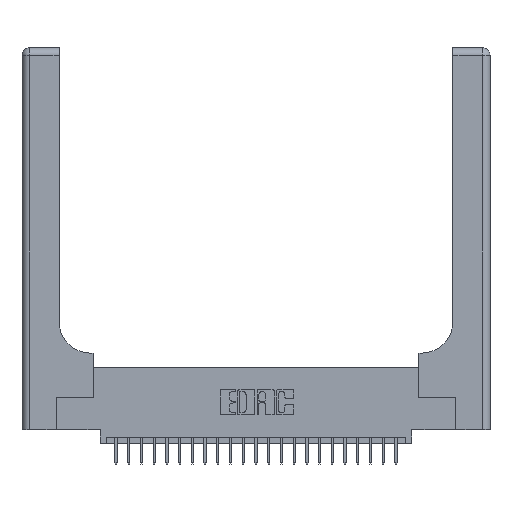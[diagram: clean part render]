
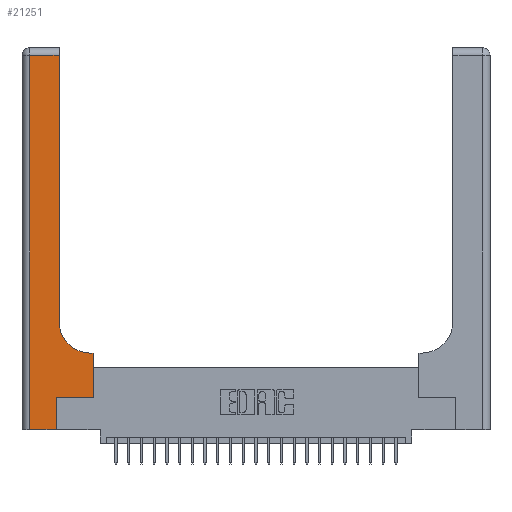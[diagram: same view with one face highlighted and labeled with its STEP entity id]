
A CAD part, top view. The second image highlights one B-rep face of the part: STEP entity #21251.
In plain terms, the highlighted planar face has unit normal (0, 0, 1).
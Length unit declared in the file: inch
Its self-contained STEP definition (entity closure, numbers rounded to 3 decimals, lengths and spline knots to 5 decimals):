
#22 = CARTESIAN_POINT ( 'NONE',  ( 0., 2.94, 0.37 ) ) ;
#69 = CARTESIAN_POINT ( 'NONE',  ( 0.5415, 0.6, 0.37 ) ) ;
#72 = DIRECTION ( 'NONE',  ( 0., 1., 0. ) ) ;
#163 = VECTOR ( 'NONE', #20187, 39.37008 ) ;
#541 = DIRECTION ( 'NONE',  ( -1., 0., 0. ) ) ;
#1038 = ORIENTED_EDGE ( 'NONE', *, *, #2842, .T. ) ;
#1463 = DIRECTION ( 'NONE',  ( -1., 0., 0. ) ) ;
#1964 = VERTEX_POINT ( 'NONE', #22152 ) ;
#2153 = CIRCLE ( 'NONE', #24305, 0.25 ) ;
#2842 = EDGE_CURVE ( 'NONE', #4173, #8693, #6901, .T. ) ;
#2894 = ORIENTED_EDGE ( 'NONE', *, *, #9883, .T. ) ;
#3102 = CARTESIAN_POINT ( 'NONE',  ( 0.5585, 0.6, 0.37 ) ) ;
#3452 = CARTESIAN_POINT ( 'NONE',  ( 0.2915, 2.94, 0.37 ) ) ;
#3675 = LINE ( 'NONE', #8064, #19081 ) ;
#3747 = EDGE_CURVE ( 'NONE', #8693, #5910, #2153, .T. ) ;
#3806 = LINE ( 'NONE', #5872, #9126 ) ;
#3822 = DIRECTION ( 'NONE',  ( 0., 0., -1. ) ) ;
#3873 = CARTESIAN_POINT ( 'NONE',  ( 0.269, 0.25, 0.37 ) ) ;
#4002 = CARTESIAN_POINT ( 'NONE',  ( 0.269, 0.25, 0.37 ) ) ;
#4028 = LINE ( 'NONE', #9681, #24755 ) ;
#4173 = VERTEX_POINT ( 'NONE', #3102 ) ;
#4700 = AXIS2_PLACEMENT_3D ( 'NONE', #17482, #13524, #1463 ) ;
#5420 = PLANE ( 'NONE',  #4700 ) ;
#5673 = EDGE_CURVE ( 'NONE', #20346, #1964, #22833, .T. ) ;
#5684 = VECTOR ( 'NONE', #18078, 39.37008 ) ;
#5872 = CARTESIAN_POINT ( 'NONE',  ( 0.269, 0., 0.37 ) ) ;
#5910 = VERTEX_POINT ( 'NONE', #7202 ) ;
#6901 = LINE ( 'NONE', #12598, #16997 ) ;
#7202 = CARTESIAN_POINT ( 'NONE',  ( 0.2915, 0.85, 0.37 ) ) ;
#7271 = VERTEX_POINT ( 'NONE', #9539 ) ;
#7895 = DIRECTION ( 'NONE',  ( 0., 1., 0. ) ) ;
#8064 = CARTESIAN_POINT ( 'NONE',  ( 0.5585, 0.25, 0.37 ) ) ;
#8371 = EDGE_LOOP ( 'NONE', ( #18967, #16104, #18759, #2894, #17577, #18590, #15262, #1038, #13385 ) ) ;
#8651 = VECTOR ( 'NONE', #15869, 39.37008 ) ;
#8693 = VERTEX_POINT ( 'NONE', #69 ) ;
#9126 = VECTOR ( 'NONE', #7895, 39.37008 ) ;
#9323 = LINE ( 'NONE', #13448, #10606 ) ;
#9409 = EDGE_CURVE ( 'NONE', #1964, #16389, #4028, .T. ) ;
#9539 = CARTESIAN_POINT ( 'NONE',  ( 0.269, 0., 0.37 ) ) ;
#9681 = CARTESIAN_POINT ( 'NONE',  ( 0.06, 3., 0.37 ) ) ;
#9883 = EDGE_CURVE ( 'NONE', #16389, #7271, #9323, .T. ) ;
#10081 = EDGE_CURVE ( 'NONE', #23888, #4173, #3675, .T. ) ;
#10606 = VECTOR ( 'NONE', #17494, 39.37008 ) ;
#12598 = CARTESIAN_POINT ( 'NONE',  ( 0.2915, 0.6, 0.37 ) ) ;
#13385 = ORIENTED_EDGE ( 'NONE', *, *, #3747, .T. ) ;
#13448 = CARTESIAN_POINT ( 'NONE',  ( 0., 0., 0.37 ) ) ;
#13524 = DIRECTION ( 'NONE',  ( 0., 0., -1. ) ) ;
#14207 = FACE_OUTER_BOUND ( 'NONE', #8371, .T. ) ;
#14482 = VERTEX_POINT ( 'NONE', #3873 ) ;
#15262 = ORIENTED_EDGE ( 'NONE', *, *, #10081, .T. ) ;
#15650 = EDGE_CURVE ( 'NONE', #14482, #23888, #25793, .T. ) ;
#15838 = CARTESIAN_POINT ( 'NONE',  ( 0.5415, 0.85, 0.37 ) ) ;
#15869 = DIRECTION ( 'NONE',  ( 0., 1., 0. ) ) ;
#16104 = ORIENTED_EDGE ( 'NONE', *, *, #5673, .T. ) ;
#16183 = EDGE_CURVE ( 'NONE', #7271, #14482, #3806, .T. ) ;
#16389 = VERTEX_POINT ( 'NONE', #22778 ) ;
#16997 = VECTOR ( 'NONE', #541, 39.37008 ) ;
#17482 = CARTESIAN_POINT ( 'NONE',  ( 0., 3., 0.37 ) ) ;
#17494 = DIRECTION ( 'NONE',  ( 1., 0., 0. ) ) ;
#17577 = ORIENTED_EDGE ( 'NONE', *, *, #16183, .T. ) ;
#17893 = DIRECTION ( 'NONE',  ( 1., 0., 0. ) ) ;
#18078 = DIRECTION ( 'NONE',  ( 1., 0., 0. ) ) ;
#18590 = ORIENTED_EDGE ( 'NONE', *, *, #15650, .T. ) ;
#18759 = ORIENTED_EDGE ( 'NONE', *, *, #9409, .T. ) ;
#18967 = ORIENTED_EDGE ( 'NONE', *, *, #19170, .T. ) ;
#19081 = VECTOR ( 'NONE', #72, 39.37008 ) ;
#19170 = EDGE_CURVE ( 'NONE', #5910, #20346, #20017, .T. ) ;
#19944 = CARTESIAN_POINT ( 'NONE',  ( 0.5585, 0.25, 0.37 ) ) ;
#20017 = LINE ( 'NONE', #21979, #8651 ) ;
#20187 = DIRECTION ( 'NONE',  ( -1., 0., 0. ) ) ;
#20346 = VERTEX_POINT ( 'NONE', #3452 ) ;
#21251 = ADVANCED_FACE ( 'NONE', ( #14207 ), #5420, .F. ) ;
#21979 = CARTESIAN_POINT ( 'NONE',  ( 0.2915, 3., 0.37 ) ) ;
#22152 = CARTESIAN_POINT ( 'NONE',  ( 0.06, 2.94, 0.37 ) ) ;
#22778 = CARTESIAN_POINT ( 'NONE',  ( 0.06, 0., 0.37 ) ) ;
#22833 = LINE ( 'NONE', #22, #163 ) ;
#23888 = VERTEX_POINT ( 'NONE', #19944 ) ;
#24305 = AXIS2_PLACEMENT_3D ( 'NONE', #15838, #3822, #17893 ) ;
#24755 = VECTOR ( 'NONE', #25738, 39.37008 ) ;
#25738 = DIRECTION ( 'NONE',  ( 0., -1., 0. ) ) ;
#25793 = LINE ( 'NONE', #4002, #5684 ) ;
